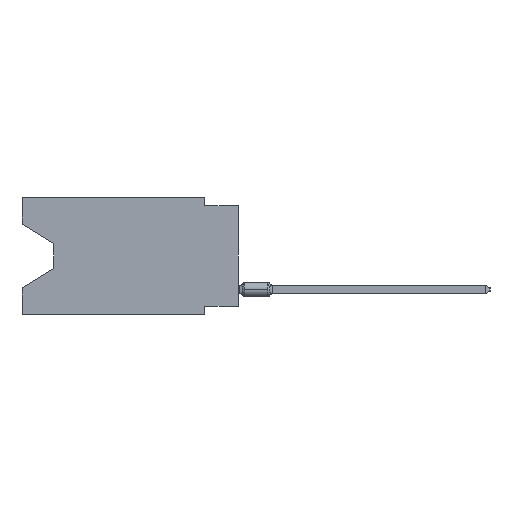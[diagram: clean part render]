
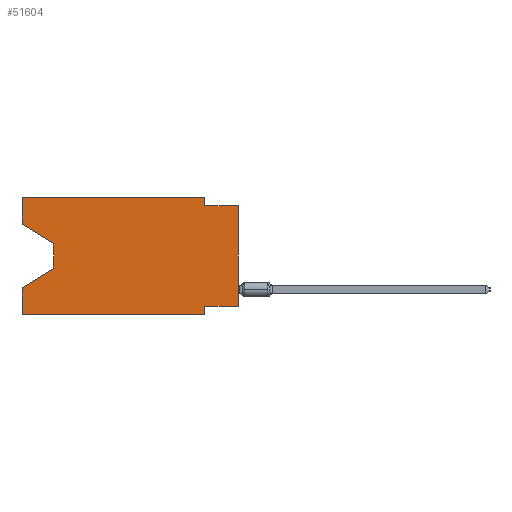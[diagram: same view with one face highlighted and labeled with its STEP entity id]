
A CAD part, left-side view. The second image highlights one B-rep face of the part: STEP entity #51604.
In plain terms, the highlighted planar face has unit normal (-1, 0, 0).
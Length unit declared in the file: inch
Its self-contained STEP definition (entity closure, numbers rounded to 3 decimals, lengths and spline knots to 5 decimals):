
#245 = VERTEX_POINT ( 'NONE', #54120 ) ;
#977 = DIRECTION ( 'NONE',  ( 0., 0., -1. ) ) ;
#1077 = LINE ( 'NONE', #22916, #68402 ) ;
#1122 = ORIENTED_EDGE ( 'NONE', *, *, #40339, .T. ) ;
#1735 = VERTEX_POINT ( 'NONE', #55182 ) ;
#2743 = VECTOR ( 'NONE', #54281, 39.37008 ) ;
#4043 = CARTESIAN_POINT ( 'NONE',  ( 0., 0.645, -0.35 ) ) ;
#4216 = DIRECTION ( 'NONE',  ( 0., 1., 0. ) ) ;
#4570 = LINE ( 'NONE', #26372, #34823 ) ;
#5107 = VERTEX_POINT ( 'NONE', #43151 ) ;
#5602 = LINE ( 'NONE', #16695, #70662 ) ;
#7720 = VERTEX_POINT ( 'NONE', #29198 ) ;
#8370 = EDGE_CURVE ( 'NONE', #7720, #245, #27639, .T. ) ;
#8435 = CARTESIAN_POINT ( 'NONE',  ( 0., 0.1, -0.325 ) ) ;
#10087 = VERTEX_POINT ( 'NONE', #57273 ) ;
#10313 = CARTESIAN_POINT ( 'NONE',  ( 0., 0.1, 0. ) ) ;
#10991 = VECTOR ( 'NONE', #32323, 39.37008 ) ;
#11625 = CARTESIAN_POINT ( 'NONE',  ( 0., 0.645, 0. ) ) ;
#14854 = EDGE_CURVE ( 'NONE', #27911, #35633, #48074, .T. ) ;
#15506 = EDGE_CURVE ( 'NONE', #5107, #51251, #1077, .T. ) ;
#15535 = ORIENTED_EDGE ( 'NONE', *, *, #62653, .F. ) ;
#16695 = CARTESIAN_POINT ( 'NONE',  ( 0., 0.55, -0.138 ) ) ;
#18235 = ORIENTED_EDGE ( 'NONE', *, *, #34735, .T. ) ;
#18995 = EDGE_CURVE ( 'NONE', #28972, #245, #32109, .T. ) ;
#20147 = LINE ( 'NONE', #4043, #33836 ) ;
#21436 = VERTEX_POINT ( 'NONE', #21933 ) ;
#21933 = CARTESIAN_POINT ( 'NONE',  ( 0., 0.55, -0.138 ) ) ;
#22559 = VECTOR ( 'NONE', #30832, 39.37008 ) ;
#22916 = CARTESIAN_POINT ( 'NONE',  ( 0., 0., -0.025 ) ) ;
#23629 = VERTEX_POINT ( 'NONE', #8435 ) ;
#23687 = CARTESIAN_POINT ( 'NONE',  ( 0., 0.645, -0.35 ) ) ;
#24626 = CARTESIAN_POINT ( 'NONE',  ( 0., 0., -0.025 ) ) ;
#24911 = ORIENTED_EDGE ( 'NONE', *, *, #8370, .T. ) ;
#26228 = CARTESIAN_POINT ( 'NONE',  ( 0., 0.55, -0.212 ) ) ;
#26372 = CARTESIAN_POINT ( 'NONE',  ( 0., 0., -0.325 ) ) ;
#27107 = DIRECTION ( 'NONE',  ( 0., 0., -1. ) ) ;
#27639 = LINE ( 'NONE', #26228, #47728 ) ;
#27911 = VERTEX_POINT ( 'NONE', #47502 ) ;
#28818 = ORIENTED_EDGE ( 'NONE', *, *, #68051, .T. ) ;
#28972 = VERTEX_POINT ( 'NONE', #23687 ) ;
#29198 = CARTESIAN_POINT ( 'NONE',  ( 0., 0.55, -0.212 ) ) ;
#30832 = DIRECTION ( 'NONE',  ( 0., -0.855, -0.519 ) ) ;
#30837 = LINE ( 'NONE', #68067, #64448 ) ;
#31947 = CARTESIAN_POINT ( 'NONE',  ( 0., 0.645, 0. ) ) ;
#32109 = LINE ( 'NONE', #53923, #2743 ) ;
#32323 = DIRECTION ( 'NONE',  ( 0., 0., 1. ) ) ;
#32337 = EDGE_CURVE ( 'NONE', #59786, #5107, #30837, .T. ) ;
#33444 = VECTOR ( 'NONE', #44583, 39.37008 ) ;
#33675 = EDGE_CURVE ( 'NONE', #1735, #23629, #4570, .T. ) ;
#33836 = VECTOR ( 'NONE', #48376, 39.37008 ) ;
#34735 = EDGE_CURVE ( 'NONE', #1735, #51251, #59529, .T. ) ;
#34823 = VECTOR ( 'NONE', #4216, 39.37008 ) ;
#34912 = AXIS2_PLACEMENT_3D ( 'NONE', #49967, #43540, #977 ) ;
#35506 = DIRECTION ( 'NONE',  ( 0., 0., -1. ) ) ;
#35633 = VERTEX_POINT ( 'NONE', #11625 ) ;
#37407 = ORIENTED_EDGE ( 'NONE', *, *, #15506, .F. ) ;
#37599 = VECTOR ( 'NONE', #27107, 39.37008 ) ;
#38611 = ORIENTED_EDGE ( 'NONE', *, *, #41076, .F. ) ;
#38845 = DIRECTION ( 'NONE',  ( 0., 0., -1. ) ) ;
#38854 = LINE ( 'NONE', #39206, #33444 ) ;
#39206 = CARTESIAN_POINT ( 'NONE',  ( 0., 0.645, 0. ) ) ;
#40339 = EDGE_CURVE ( 'NONE', #21436, #7720, #5602, .T. ) ;
#40496 = ORIENTED_EDGE ( 'NONE', *, *, #32337, .F. ) ;
#41076 = EDGE_CURVE ( 'NONE', #23629, #10087, #64674, .T. ) ;
#41989 = DIRECTION ( 'NONE',  ( 0., 0., 1. ) ) ;
#43151 = CARTESIAN_POINT ( 'NONE',  ( 0., 0.1, -0.025 ) ) ;
#43486 = ORIENTED_EDGE ( 'NONE', *, *, #14854, .F. ) ;
#43540 = DIRECTION ( 'NONE',  ( 1., 0., 0. ) ) ;
#43882 = FACE_OUTER_BOUND ( 'NONE', #55500, .T. ) ;
#44583 = DIRECTION ( 'NONE',  ( 0., -1., 0. ) ) ;
#44698 = DIRECTION ( 'NONE',  ( 0., -1., 0. ) ) ;
#47502 = CARTESIAN_POINT ( 'NONE',  ( 0., 0.645, -0.08025 ) ) ;
#47728 = VECTOR ( 'NONE', #48392, 39.37008 ) ;
#48074 = LINE ( 'NONE', #31947, #50036 ) ;
#48376 = DIRECTION ( 'NONE',  ( 0., -1., 0. ) ) ;
#48392 = DIRECTION ( 'NONE',  ( 0., 0.855, -0.519 ) ) ;
#49967 = CARTESIAN_POINT ( 'NONE',  ( 0., 0.645, 0. ) ) ;
#50036 = VECTOR ( 'NONE', #41989, 39.37008 ) ;
#50925 = ORIENTED_EDGE ( 'NONE', *, *, #18995, .F. ) ;
#51251 = VERTEX_POINT ( 'NONE', #24626 ) ;
#51604 = ADVANCED_FACE ( 'NONE', ( #43882 ), #56036, .F. ) ;
#52290 = CARTESIAN_POINT ( 'NONE',  ( 0., 0.645, -0.08025 ) ) ;
#53923 = CARTESIAN_POINT ( 'NONE',  ( 0., 0.645, 0. ) ) ;
#54120 = CARTESIAN_POINT ( 'NONE',  ( 0., 0.645, -0.26975 ) ) ;
#54281 = DIRECTION ( 'NONE',  ( 0., 0., 1. ) ) ;
#54998 = CARTESIAN_POINT ( 'NONE',  ( 0., 0.1, -0.35 ) ) ;
#55182 = CARTESIAN_POINT ( 'NONE',  ( 0., 0., -0.325 ) ) ;
#55183 = EDGE_CURVE ( 'NONE', #27911, #21436, #63388, .T. ) ;
#55500 = EDGE_LOOP ( 'NONE', ( #55921, #1122, #24911, #50925, #28818, #38611, #61223, #18235, #37407, #40496, #15535, #43486 ) ) ;
#55921 = ORIENTED_EDGE ( 'NONE', *, *, #55183, .T. ) ;
#56036 = PLANE ( 'NONE',  #34912 ) ;
#57273 = CARTESIAN_POINT ( 'NONE',  ( 0., 0.1, -0.35 ) ) ;
#59529 = LINE ( 'NONE', #69921, #10991 ) ;
#59786 = VERTEX_POINT ( 'NONE', #10313 ) ;
#61223 = ORIENTED_EDGE ( 'NONE', *, *, #33675, .F. ) ;
#62653 = EDGE_CURVE ( 'NONE', #35633, #59786, #38854, .T. ) ;
#63388 = LINE ( 'NONE', #52290, #22559 ) ;
#64448 = VECTOR ( 'NONE', #35506, 39.37008 ) ;
#64674 = LINE ( 'NONE', #54998, #37599 ) ;
#68051 = EDGE_CURVE ( 'NONE', #28972, #10087, #20147, .T. ) ;
#68067 = CARTESIAN_POINT ( 'NONE',  ( 0., 0.1, 0. ) ) ;
#68402 = VECTOR ( 'NONE', #44698, 39.37008 ) ;
#69921 = CARTESIAN_POINT ( 'NONE',  ( 0., 0., 0. ) ) ;
#70662 = VECTOR ( 'NONE', #38845, 39.37008 ) ;
